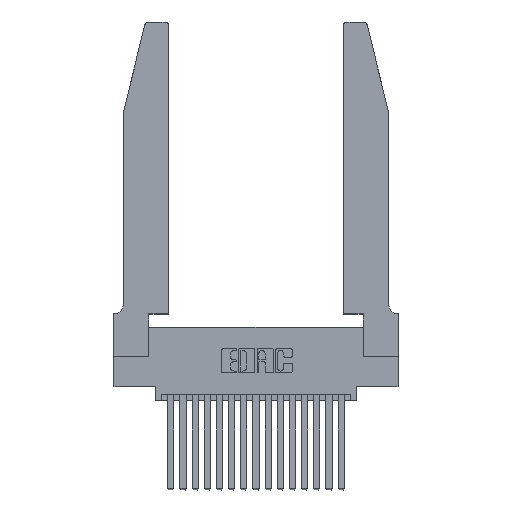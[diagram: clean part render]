
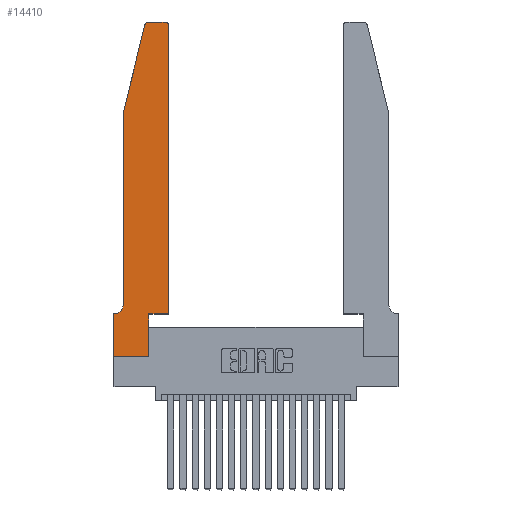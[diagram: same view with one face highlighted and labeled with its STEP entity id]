
A CAD part, top view. The second image highlights one B-rep face of the part: STEP entity #14410.
In plain terms, the highlighted planar face has unit normal (0, 0, 1).
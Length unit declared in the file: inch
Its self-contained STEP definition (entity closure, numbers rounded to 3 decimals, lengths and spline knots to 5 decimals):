
#111 = CARTESIAN_POINT ( 'NONE',  ( 0.0755, 2., 0.37 ) ) ;
#266 = CARTESIAN_POINT ( 'NONE',  ( 0., 0., 0.37 ) ) ;
#425 = VERTEX_POINT ( 'NONE', #3109 ) ;
#512 = EDGE_CURVE ( 'NONE', #17260, #14690, #17694, .T. ) ;
#545 = VECTOR ( 'NONE', #12090, 39.37008 ) ;
#820 = EDGE_CURVE ( 'NONE', #14690, #18094, #11115, .T. ) ;
#1162 = CARTESIAN_POINT ( 'NONE',  ( 0.0755, 0.35, 0.37 ) ) ;
#1437 = DIRECTION ( 'NONE',  ( -1., 0., 0. ) ) ;
#1456 = CARTESIAN_POINT ( 'NONE',  ( 0., 0.35, 0.37 ) ) ;
#1640 = CARTESIAN_POINT ( 'NONE',  ( 0.0755, 2., 0.37 ) ) ;
#1717 = DIRECTION ( 'NONE',  ( 0., -1., 0. ) ) ;
#1984 = DIRECTION ( 'NONE',  ( -0.239, -0.971, 0. ) ) ;
#2095 = DIRECTION ( 'NONE',  ( 0., 0., -1. ) ) ;
#2168 = VERTEX_POINT ( 'NONE', #18726 ) ;
#2585 = CIRCLE ( 'NONE', #18540, 0.03 ) ;
#2683 = CARTESIAN_POINT ( 'NONE',  ( 0.4505, 0.35, 0.37 ) ) ;
#2827 = DIRECTION ( 'NONE',  ( 0., 0., 1. ) ) ;
#2842 = EDGE_CURVE ( 'NONE', #15001, #2168, #8385, .T. ) ;
#2868 = DIRECTION ( 'NONE',  ( -1., 0., 0. ) ) ;
#3109 = CARTESIAN_POINT ( 'NONE',  ( 0., 0.35, 0.37 ) ) ;
#3128 = DIRECTION ( 'NONE',  ( 1., 0., 0. ) ) ;
#3296 = DIRECTION ( 'NONE',  ( 1., 0., 0. ) ) ;
#3550 = CARTESIAN_POINT ( 'NONE',  ( 0.284, 2.72, 0.37 ) ) ;
#3583 = DIRECTION ( 'NONE',  ( 0., -1., 0. ) ) ;
#3592 = CARTESIAN_POINT ( 'NONE',  ( 0.0055, 0.42, 0.37 ) ) ;
#3648 = VECTOR ( 'NONE', #3296, 39.37008 ) ;
#3876 = EDGE_CURVE ( 'NONE', #7136, #14835, #16409, .T. ) ;
#3994 = LINE ( 'NONE', #4755, #18787 ) ;
#4320 = DIRECTION ( 'NONE',  ( 0., 1., 0. ) ) ;
#4511 = LINE ( 'NONE', #5876, #16261 ) ;
#4755 = CARTESIAN_POINT ( 'NONE',  ( 0.4505, 0.35, 0.37 ) ) ;
#5177 = DIRECTION ( 'NONE',  ( 1., 0., 0. ) ) ;
#5876 = CARTESIAN_POINT ( 'NONE',  ( 0.2865, 0.35, 0.37 ) ) ;
#6686 = ORIENTED_EDGE ( 'NONE', *, *, #820, .T. ) ;
#7136 = VERTEX_POINT ( 'NONE', #11902 ) ;
#7174 = LINE ( 'NONE', #9924, #14854 ) ;
#7207 = CIRCLE ( 'NONE', #7877, 0.03 ) ;
#7877 = AXIS2_PLACEMENT_3D ( 'NONE', #3550, #14398, #5177 ) ;
#7903 = ORIENTED_EDGE ( 'NONE', *, *, #11097, .T. ) ;
#8056 = VECTOR ( 'NONE', #3583, 39.37008 ) ;
#8377 = DIRECTION ( 'NONE',  ( 0., 1., 0. ) ) ;
#8385 = LINE ( 'NONE', #2683, #19916 ) ;
#8568 = CARTESIAN_POINT ( 'NONE',  ( 0.0755, 0.42, 0.37 ) ) ;
#8600 = LINE ( 'NONE', #266, #8056 ) ;
#8667 = EDGE_CURVE ( 'NONE', #15817, #9906, #7207, .T. ) ;
#8723 = ORIENTED_EDGE ( 'NONE', *, *, #9500, .T. ) ;
#8923 = VERTEX_POINT ( 'NONE', #10699 ) ;
#9164 = LINE ( 'NONE', #10567, #545 ) ;
#9500 = EDGE_CURVE ( 'NONE', #14835, #8923, #4511, .T. ) ;
#9906 = VERTEX_POINT ( 'NONE', #15122 ) ;
#9924 = CARTESIAN_POINT ( 'NONE',  ( 0.0755, 2., 0.37 ) ) ;
#10264 = CARTESIAN_POINT ( 'NONE',  ( 0.284, 2.75, 0.37 ) ) ;
#10279 = EDGE_CURVE ( 'NONE', #9906, #17260, #7174, .T. ) ;
#10392 = ORIENTED_EDGE ( 'NONE', *, *, #512, .T. ) ;
#10567 = CARTESIAN_POINT ( 'NONE',  ( 0.2605, 2.75, 0.37 ) ) ;
#10699 = CARTESIAN_POINT ( 'NONE',  ( 0.2865, 0.35, 0.37 ) ) ;
#10782 = EDGE_CURVE ( 'NONE', #8923, #15001, #3994, .T. ) ;
#11097 = EDGE_CURVE ( 'NONE', #12843, #15817, #9164, .T. ) ;
#11115 = CIRCLE ( 'NONE', #16334, 0.07 ) ;
#11339 = ORIENTED_EDGE ( 'NONE', *, *, #17334, .T. ) ;
#11902 = CARTESIAN_POINT ( 'NONE',  ( 0., 0., 0.37 ) ) ;
#12042 = ORIENTED_EDGE ( 'NONE', *, *, #8667, .T. ) ;
#12090 = DIRECTION ( 'NONE',  ( -1., 0., 0. ) ) ;
#12234 = CARTESIAN_POINT ( 'NONE',  ( 0.4205, 2.72, 0.37 ) ) ;
#12365 = CARTESIAN_POINT ( 'NONE',  ( 0.4505, 0.35, 0.37 ) ) ;
#12520 = DIRECTION ( 'NONE',  ( 0., 0., 1. ) ) ;
#12522 = ORIENTED_EDGE ( 'NONE', *, *, #10279, .T. ) ;
#12843 = VERTEX_POINT ( 'NONE', #16614 ) ;
#13263 = ORIENTED_EDGE ( 'NONE', *, *, #10782, .T. ) ;
#13297 = VECTOR ( 'NONE', #1717, 39.37008 ) ;
#13505 = CARTESIAN_POINT ( 'NONE',  ( 0.2865, 0., 0.37 ) ) ;
#13748 = DIRECTION ( 'NONE',  ( 1., 0., 0. ) ) ;
#14034 = LINE ( 'NONE', #1162, #16581 ) ;
#14398 = DIRECTION ( 'NONE',  ( 0., 0., 1. ) ) ;
#14410 = ADVANCED_FACE ( 'NONE', ( #18318 ), #16928, .T. ) ;
#14690 = VERTEX_POINT ( 'NONE', #8568 ) ;
#14835 = VERTEX_POINT ( 'NONE', #13505 ) ;
#14851 = ORIENTED_EDGE ( 'NONE', *, *, #17054, .T. ) ;
#14854 = VECTOR ( 'NONE', #1984, 39.37008 ) ;
#15001 = VERTEX_POINT ( 'NONE', #12365 ) ;
#15122 = CARTESIAN_POINT ( 'NONE',  ( 0.25487, 2.72718, 0.37 ) ) ;
#15138 = AXIS2_PLACEMENT_3D ( 'NONE', #1456, #12520, #3128 ) ;
#15486 = DIRECTION ( 'NONE',  ( 1., 0., 0. ) ) ;
#15817 = VERTEX_POINT ( 'NONE', #10264 ) ;
#15876 = EDGE_LOOP ( 'NONE', ( #7903, #12042, #12522, #10392, #6686, #14851, #11339, #19280, #8723, #13263, #17168, #17662 ) ) ;
#15974 = CARTESIAN_POINT ( 'NONE',  ( 0., 0., 0.37 ) ) ;
#16261 = VECTOR ( 'NONE', #4320, 39.37008 ) ;
#16334 = AXIS2_PLACEMENT_3D ( 'NONE', #3592, #2095, #1437 ) ;
#16409 = LINE ( 'NONE', #15974, #3648 ) ;
#16558 = EDGE_CURVE ( 'NONE', #2168, #12843, #2585, .T. ) ;
#16581 = VECTOR ( 'NONE', #2868, 39.37008 ) ;
#16614 = CARTESIAN_POINT ( 'NONE',  ( 0.4205, 2.75, 0.37 ) ) ;
#16928 = PLANE ( 'NONE',  #15138 ) ;
#17054 = EDGE_CURVE ( 'NONE', #18094, #425, #14034, .T. ) ;
#17168 = ORIENTED_EDGE ( 'NONE', *, *, #2842, .T. ) ;
#17260 = VERTEX_POINT ( 'NONE', #111 ) ;
#17334 = EDGE_CURVE ( 'NONE', #425, #7136, #8600, .T. ) ;
#17499 = CARTESIAN_POINT ( 'NONE',  ( 0.0055, 0.35, 0.37 ) ) ;
#17662 = ORIENTED_EDGE ( 'NONE', *, *, #16558, .T. ) ;
#17694 = LINE ( 'NONE', #1640, #13297 ) ;
#18094 = VERTEX_POINT ( 'NONE', #17499 ) ;
#18318 = FACE_OUTER_BOUND ( 'NONE', #15876, .T. ) ;
#18540 = AXIS2_PLACEMENT_3D ( 'NONE', #12234, #2827, #13748 ) ;
#18726 = CARTESIAN_POINT ( 'NONE',  ( 0.4505, 2.72, 0.37 ) ) ;
#18787 = VECTOR ( 'NONE', #15486, 39.37008 ) ;
#19280 = ORIENTED_EDGE ( 'NONE', *, *, #3876, .T. ) ;
#19916 = VECTOR ( 'NONE', #8377, 39.37008 ) ;
